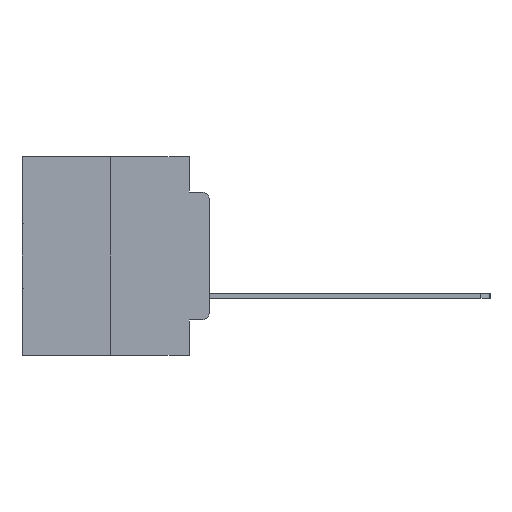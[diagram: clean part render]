
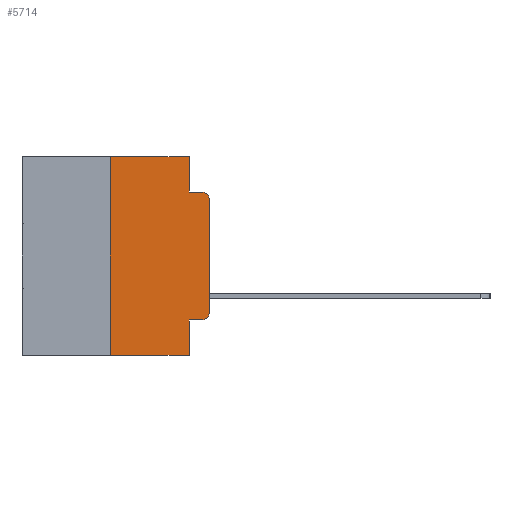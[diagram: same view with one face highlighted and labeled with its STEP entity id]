
A CAD part, left-side view. The second image highlights one B-rep face of the part: STEP entity #5714.
In plain terms, the highlighted planar face has unit normal (-1, 0, 0).
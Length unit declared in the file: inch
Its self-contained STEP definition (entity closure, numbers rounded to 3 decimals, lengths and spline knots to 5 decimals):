
#258 = CARTESIAN_POINT ( 'NONE',  ( 0., 0.051, 0. ) ) ;
#291 = VERTEX_POINT ( 'NONE', #23629 ) ;
#440 = EDGE_LOOP ( 'NONE', ( #27392, #22846, #6024, #12201, #1214, #2716, #27758, #17229, #26018, #5320 ) ) ;
#897 = LINE ( 'NONE', #258, #12631 ) ;
#1103 = DIRECTION ( 'NONE',  ( 0., -1., 0. ) ) ;
#1214 = ORIENTED_EDGE ( 'NONE', *, *, #26211, .F. ) ;
#1234 = VERTEX_POINT ( 'NONE', #13785 ) ;
#1886 = CARTESIAN_POINT ( 'NONE',  ( 0., 0.051, -0.4115 ) ) ;
#2404 = VERTEX_POINT ( 'NONE', #16109 ) ;
#2505 = LINE ( 'NONE', #1886, #19485 ) ;
#2682 = DIRECTION ( 'NONE',  ( 0., 0., -1. ) ) ;
#2707 = EDGE_CURVE ( 'NONE', #29246, #28523, #24898, .T. ) ;
#2716 = ORIENTED_EDGE ( 'NONE', *, *, #11146, .F. ) ;
#3166 = EDGE_CURVE ( 'NONE', #23617, #291, #28735, .T. ) ;
#3177 = FACE_OUTER_BOUND ( 'NONE', #440, .T. ) ;
#3495 = VERTEX_POINT ( 'NONE', #15983 ) ;
#3514 = CARTESIAN_POINT ( 'NONE',  ( 0., 0.25, 0. ) ) ;
#4227 = CARTESIAN_POINT ( 'NONE',  ( 0., 0.02, -0.4115 ) ) ;
#4242 = DIRECTION ( 'NONE',  ( 0., -1., 0. ) ) ;
#4940 = DIRECTION ( 'NONE',  ( 0., -1., 0. ) ) ;
#5206 = VECTOR ( 'NONE', #13913, 39.37008 ) ;
#5320 = ORIENTED_EDGE ( 'NONE', *, *, #3166, .T. ) ;
#5714 = ADVANCED_FACE ( 'NONE', ( #3177 ), #26368, .F. ) ;
#6024 = ORIENTED_EDGE ( 'NONE', *, *, #2707, .F. ) ;
#6700 = VECTOR ( 'NONE', #25015, 39.37008 ) ;
#7101 = DIRECTION ( 'NONE',  ( 0., 0., 1. ) ) ;
#7174 = AXIS2_PLACEMENT_3D ( 'NONE', #25230, #11662, #27474 ) ;
#7887 = VERTEX_POINT ( 'NONE', #3514 ) ;
#8203 = AXIS2_PLACEMENT_3D ( 'NONE', #25372, #26727, #27499 ) ;
#8598 = LINE ( 'NONE', #19641, #20711 ) ;
#8825 = LINE ( 'NONE', #23073, #14208 ) ;
#9452 = LINE ( 'NONE', #18737, #27498 ) ;
#10582 = EDGE_CURVE ( 'NONE', #2404, #28523, #11582, .T. ) ;
#10634 = EDGE_CURVE ( 'NONE', #15001, #23571, #9452, .T. ) ;
#11146 = EDGE_CURVE ( 'NONE', #15001, #7887, #25365, .T. ) ;
#11582 = CIRCLE ( 'NONE', #7174, 0.02 ) ;
#11662 = DIRECTION ( 'NONE',  ( -1., 0., 0. ) ) ;
#12201 = ORIENTED_EDGE ( 'NONE', *, *, #27797, .F. ) ;
#12631 = VECTOR ( 'NONE', #2682, 39.37008 ) ;
#12929 = DIRECTION ( 'NONE',  ( 0., 0., -1. ) ) ;
#13785 = CARTESIAN_POINT ( 'NONE',  ( 0., 0.051, 0. ) ) ;
#13829 = CARTESIAN_POINT ( 'NONE',  ( 0., 0.25, 0. ) ) ;
#13913 = DIRECTION ( 'NONE',  ( 0., 0., -1. ) ) ;
#14208 = VECTOR ( 'NONE', #7101, 39.37008 ) ;
#15001 = VERTEX_POINT ( 'NONE', #17188 ) ;
#15983 = CARTESIAN_POINT ( 'NONE',  ( 0., 0.051, -0.4115 ) ) ;
#16109 = CARTESIAN_POINT ( 'NONE',  ( 0., 0., -0.1085 ) ) ;
#17148 = EDGE_CURVE ( 'NONE', #3495, #23617, #2505, .T. ) ;
#17188 = CARTESIAN_POINT ( 'NONE',  ( 0., 0.25, -0.5 ) ) ;
#17229 = ORIENTED_EDGE ( 'NONE', *, *, #18471, .F. ) ;
#18471 = EDGE_CURVE ( 'NONE', #3495, #23571, #897, .T. ) ;
#18488 = CARTESIAN_POINT ( 'NONE',  ( 0., 0.051, 0. ) ) ;
#18737 = CARTESIAN_POINT ( 'NONE',  ( 0., 0.473, -0.5 ) ) ;
#19485 = VECTOR ( 'NONE', #4242, 39.37008 ) ;
#19641 = CARTESIAN_POINT ( 'NONE',  ( 0., 0.473, 0. ) ) ;
#19703 = CARTESIAN_POINT ( 'NONE',  ( 0., 0.473, 0. ) ) ;
#20247 = CARTESIAN_POINT ( 'NONE',  ( 0., 0.051, -0.5 ) ) ;
#20711 = VECTOR ( 'NONE', #1103, 39.37008 ) ;
#21023 = CARTESIAN_POINT ( 'NONE',  ( 0., 0.02, -0.0885 ) ) ;
#22846 = ORIENTED_EDGE ( 'NONE', *, *, #10582, .T. ) ;
#23073 = CARTESIAN_POINT ( 'NONE',  ( 0., 0., 0. ) ) ;
#23524 = AXIS2_PLACEMENT_3D ( 'NONE', #19703, #26466, #12929 ) ;
#23571 = VERTEX_POINT ( 'NONE', #20247 ) ;
#23617 = VERTEX_POINT ( 'NONE', #4227 ) ;
#23629 = CARTESIAN_POINT ( 'NONE',  ( 0., 0., -0.3915 ) ) ;
#24675 = VECTOR ( 'NONE', #25097, 39.37008 ) ;
#24898 = LINE ( 'NONE', #25537, #6700 ) ;
#25015 = DIRECTION ( 'NONE',  ( 0., -1., 0. ) ) ;
#25097 = DIRECTION ( 'NONE',  ( 0., 0., 1. ) ) ;
#25230 = CARTESIAN_POINT ( 'NONE',  ( 0., 0.02, -0.1085 ) ) ;
#25365 = LINE ( 'NONE', #13829, #24675 ) ;
#25372 = CARTESIAN_POINT ( 'NONE',  ( 0., 0.02, -0.3915 ) ) ;
#25537 = CARTESIAN_POINT ( 'NONE',  ( 0., 0.051, -0.0885 ) ) ;
#26018 = ORIENTED_EDGE ( 'NONE', *, *, #17148, .T. ) ;
#26211 = EDGE_CURVE ( 'NONE', #7887, #1234, #8598, .T. ) ;
#26368 = PLANE ( 'NONE',  #23524 ) ;
#26466 = DIRECTION ( 'NONE',  ( 1., 0., 0. ) ) ;
#26727 = DIRECTION ( 'NONE',  ( -1., 0., 0. ) ) ;
#27392 = ORIENTED_EDGE ( 'NONE', *, *, #28993, .T. ) ;
#27474 = DIRECTION ( 'NONE',  ( 0., 0., -1. ) ) ;
#27498 = VECTOR ( 'NONE', #4940, 39.37008 ) ;
#27499 = DIRECTION ( 'NONE',  ( 0., 0., -1. ) ) ;
#27758 = ORIENTED_EDGE ( 'NONE', *, *, #10634, .T. ) ;
#27797 = EDGE_CURVE ( 'NONE', #1234, #29246, #29466, .T. ) ;
#28446 = CARTESIAN_POINT ( 'NONE',  ( 0., 0.051, -0.0885 ) ) ;
#28523 = VERTEX_POINT ( 'NONE', #21023 ) ;
#28735 = CIRCLE ( 'NONE', #8203, 0.02 ) ;
#28993 = EDGE_CURVE ( 'NONE', #291, #2404, #8825, .T. ) ;
#29246 = VERTEX_POINT ( 'NONE', #28446 ) ;
#29466 = LINE ( 'NONE', #18488, #5206 ) ;
